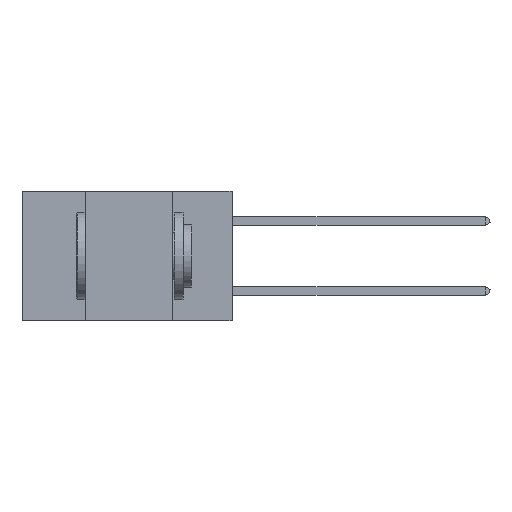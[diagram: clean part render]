
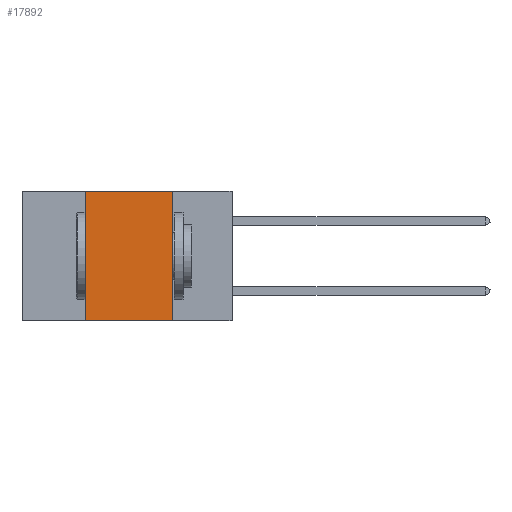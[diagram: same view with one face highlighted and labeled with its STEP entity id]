
A CAD part, left-side view. The second image highlights one B-rep face of the part: STEP entity #17892.
In plain terms, the highlighted planar face has unit normal (-1, 0, 0).
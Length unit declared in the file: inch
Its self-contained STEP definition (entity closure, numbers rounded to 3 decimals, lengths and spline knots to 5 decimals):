
#417 = ORIENTED_EDGE ( 'NONE', *, *, #24383, .F. ) ;
#435 = FACE_OUTER_BOUND ( 'NONE', #34334, .T. ) ;
#1760 = VECTOR ( 'NONE', #33296, 39.37008 ) ;
#3089 = LINE ( 'NONE', #16762, #4053 ) ;
#4053 = VECTOR ( 'NONE', #38177, 39.37008 ) ;
#4313 = ORIENTED_EDGE ( 'NONE', *, *, #13913, .F. ) ;
#5925 = CARTESIAN_POINT ( 'NONE',  ( 0., 0.6, 0. ) ) ;
#5971 = VERTEX_POINT ( 'NONE', #17106 ) ;
#6401 = CARTESIAN_POINT ( 'NONE',  ( 0., 0.6, -0.37 ) ) ;
#8076 = ORIENTED_EDGE ( 'NONE', *, *, #29925, .F. ) ;
#8146 = DIRECTION ( 'NONE',  ( 0., 0., 1. ) ) ;
#8938 = LINE ( 'NONE', #6401, #1760 ) ;
#10019 = CARTESIAN_POINT ( 'NONE',  ( 0., 0.17, 0. ) ) ;
#12904 = EDGE_CURVE ( 'NONE', #5971, #37824, #8938, .T. ) ;
#13580 = VERTEX_POINT ( 'NONE', #32984 ) ;
#13913 = EDGE_CURVE ( 'NONE', #23192, #13580, #3089, .T. ) ;
#15951 = LINE ( 'NONE', #10019, #30251 ) ;
#16762 = CARTESIAN_POINT ( 'NONE',  ( 0., 0.6, 0. ) ) ;
#17106 = CARTESIAN_POINT ( 'NONE',  ( 0., 0.42, -0.37 ) ) ;
#17892 = ADVANCED_FACE ( 'NONE', ( #435 ), #26735, .F. ) ;
#20039 = ORIENTED_EDGE ( 'NONE', *, *, #12904, .T. ) ;
#21094 = LINE ( 'NONE', #29102, #33116 ) ;
#21427 = CARTESIAN_POINT ( 'NONE',  ( 0., 0.42, 0. ) ) ;
#23192 = VERTEX_POINT ( 'NONE', #21427 ) ;
#24383 = EDGE_CURVE ( 'NONE', #5971, #23192, #21094, .T. ) ;
#25745 = CARTESIAN_POINT ( 'NONE',  ( 0., 0.17, -0.37 ) ) ;
#26685 = AXIS2_PLACEMENT_3D ( 'NONE', #5925, #27261, #35990 ) ;
#26735 = PLANE ( 'NONE',  #26685 ) ;
#27261 = DIRECTION ( 'NONE',  ( 1., 0., 0. ) ) ;
#29102 = CARTESIAN_POINT ( 'NONE',  ( 0., 0.42, 0. ) ) ;
#29925 = EDGE_CURVE ( 'NONE', #13580, #37824, #15951, .T. ) ;
#30251 = VECTOR ( 'NONE', #31132, 39.37008 ) ;
#31132 = DIRECTION ( 'NONE',  ( 0., 0., -1. ) ) ;
#32984 = CARTESIAN_POINT ( 'NONE',  ( 0., 0.17, 0. ) ) ;
#33116 = VECTOR ( 'NONE', #8146, 39.37008 ) ;
#33296 = DIRECTION ( 'NONE',  ( 0., -1., 0. ) ) ;
#34334 = EDGE_LOOP ( 'NONE', ( #8076, #4313, #417, #20039 ) ) ;
#35990 = DIRECTION ( 'NONE',  ( 0., 0., -1. ) ) ;
#37824 = VERTEX_POINT ( 'NONE', #25745 ) ;
#38177 = DIRECTION ( 'NONE',  ( 0., -1., 0. ) ) ;
